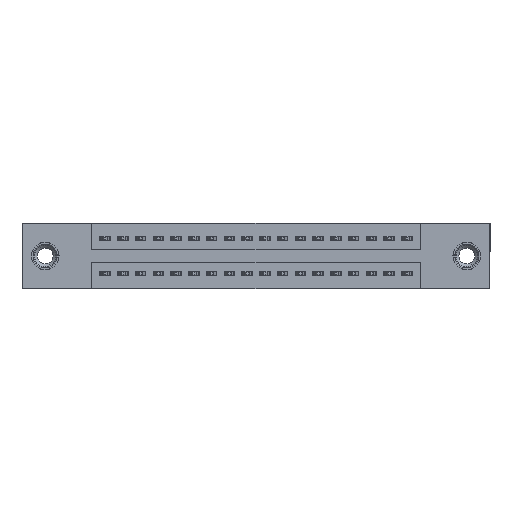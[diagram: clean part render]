
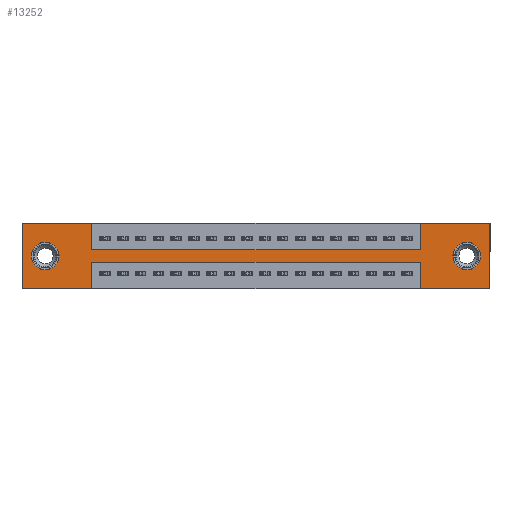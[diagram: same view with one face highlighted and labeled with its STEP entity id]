
A CAD part, front view. The second image highlights one B-rep face of the part: STEP entity #13252.
In plain terms, the highlighted planar face has unit normal (0, -1, 0).
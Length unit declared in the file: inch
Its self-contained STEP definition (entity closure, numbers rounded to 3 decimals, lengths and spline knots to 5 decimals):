
#41 = EDGE_LOOP ( 'NONE', ( #4780, #4870, #1820, #1721, #2063, #2196, #6048, #524, #962, #1680, #601, #4953 ) ) ;
#108 = EDGE_LOOP ( 'NONE', ( #6852, #15139 ) ) ;
#152 = VECTOR ( 'NONE', #4860, 39.37008 ) ;
#318 = CARTESIAN_POINT ( 'NONE',  ( 2.635, 0., -0.37 ) ) ;
#524 = ORIENTED_EDGE ( 'NONE', *, *, #14031, .F. ) ;
#582 = LINE ( 'NONE', #17118, #8273 ) ;
#601 = ORIENTED_EDGE ( 'NONE', *, *, #5658, .F. ) ;
#962 = ORIENTED_EDGE ( 'NONE', *, *, #12562, .F. ) ;
#1312 = CARTESIAN_POINT ( 'NONE',  ( 0.3925, 0., -0.37 ) ) ;
#1385 = DIRECTION ( 'NONE',  ( 0., 0., -1. ) ) ;
#1387 = DIRECTION ( 'NONE',  ( 0., 0., -1. ) ) ;
#1504 = DIRECTION ( 'NONE',  ( 0., 0., -1. ) ) ;
#1521 = DIRECTION ( 'NONE',  ( -1., 0., 0. ) ) ;
#1533 = VECTOR ( 'NONE', #14703, 39.37008 ) ;
#1588 = CIRCLE ( 'NONE', #16197, 0.078 ) ;
#1680 = ORIENTED_EDGE ( 'NONE', *, *, #13107, .F. ) ;
#1721 = ORIENTED_EDGE ( 'NONE', *, *, #17883, .F. ) ;
#1820 = ORIENTED_EDGE ( 'NONE', *, *, #15343, .F. ) ;
#1872 = CARTESIAN_POINT ( 'NONE',  ( 0., 0., 0. ) ) ;
#2063 = ORIENTED_EDGE ( 'NONE', *, *, #8920, .F. ) ;
#2196 = ORIENTED_EDGE ( 'NONE', *, *, #2887, .F. ) ;
#2735 = VERTEX_POINT ( 'NONE', #13719 ) ;
#2766 = DIRECTION ( 'NONE',  ( 1., 0., 0. ) ) ;
#2886 = VECTOR ( 'NONE', #1521, 39.37008 ) ;
#2887 = EDGE_CURVE ( 'NONE', #11552, #13812, #14918, .T. ) ;
#3115 = EDGE_LOOP ( 'NONE', ( #5435, #9566 ) ) ;
#3191 = EDGE_CURVE ( 'NONE', #7550, #15297, #17649, .T. ) ;
#3318 = VECTOR ( 'NONE', #1504, 39.37008 ) ;
#3362 = VERTEX_POINT ( 'NONE', #9424 ) ;
#3651 = CARTESIAN_POINT ( 'NONE',  ( 0.13, 0., -0.185 ) ) ;
#3683 = CARTESIAN_POINT ( 'NONE',  ( 0., 0., -0.37 ) ) ;
#4094 = VERTEX_POINT ( 'NONE', #15464 ) ;
#4113 = CARTESIAN_POINT ( 'NONE',  ( 0., 0., 0. ) ) ;
#4128 = VERTEX_POINT ( 'NONE', #14123 ) ;
#4216 = AXIS2_PLACEMENT_3D ( 'NONE', #10739, #6169, #16668 ) ;
#4217 = CARTESIAN_POINT ( 'NONE',  ( 2.635, 0., 0. ) ) ;
#4353 = CARTESIAN_POINT ( 'NONE',  ( 2.635, 0., 0. ) ) ;
#4401 = CARTESIAN_POINT ( 'NONE',  ( 2.2425, 0., -0.22 ) ) ;
#4633 = PLANE ( 'NONE',  #4216 ) ;
#4780 = ORIENTED_EDGE ( 'NONE', *, *, #16387, .F. ) ;
#4860 = DIRECTION ( 'NONE',  ( 1., 0., 0. ) ) ;
#4870 = ORIENTED_EDGE ( 'NONE', *, *, #10875, .F. ) ;
#4953 = ORIENTED_EDGE ( 'NONE', *, *, #16055, .F. ) ;
#5014 = CARTESIAN_POINT ( 'NONE',  ( 2.505, 0., -0.107 ) ) ;
#5093 = VERTEX_POINT ( 'NONE', #4401 ) ;
#5167 = DIRECTION ( 'NONE',  ( 0., 0., 1. ) ) ;
#5435 = ORIENTED_EDGE ( 'NONE', *, *, #14413, .T. ) ;
#5601 = LINE ( 'NONE', #4113, #1533 ) ;
#5604 = AXIS2_PLACEMENT_3D ( 'NONE', #8463, #18890, #10000 ) ;
#5658 = EDGE_CURVE ( 'NONE', #4128, #2735, #5601, .T. ) ;
#5840 = CARTESIAN_POINT ( 'NONE',  ( 0., 0., 0. ) ) ;
#5999 = CARTESIAN_POINT ( 'NONE',  ( 0.3925, 0., -0.37 ) ) ;
#6048 = ORIENTED_EDGE ( 'NONE', *, *, #18823, .F. ) ;
#6169 = DIRECTION ( 'NONE',  ( 0., -1., 0. ) ) ;
#6553 = VECTOR ( 'NONE', #11298, 39.37008 ) ;
#6793 = DIRECTION ( 'NONE',  ( 0., 0., 1. ) ) ;
#6852 = ORIENTED_EDGE ( 'NONE', *, *, #9925, .T. ) ;
#7401 = LINE ( 'NONE', #13758, #3318 ) ;
#7550 = VERTEX_POINT ( 'NONE', #8670 ) ;
#7720 = CARTESIAN_POINT ( 'NONE',  ( 2.2425, 0., -0.15 ) ) ;
#8029 = AXIS2_PLACEMENT_3D ( 'NONE', #3651, #14250, #5167 ) ;
#8048 = CARTESIAN_POINT ( 'NONE',  ( 0.3925, 0., -0.15 ) ) ;
#8273 = VECTOR ( 'NONE', #18610, 39.37008 ) ;
#8451 = VERTEX_POINT ( 'NONE', #7720 ) ;
#8463 = CARTESIAN_POINT ( 'NONE',  ( 0.13, 0., -0.185 ) ) ;
#8566 = VERTEX_POINT ( 'NONE', #318 ) ;
#8630 = LINE ( 'NONE', #4217, #16094 ) ;
#8670 = CARTESIAN_POINT ( 'NONE',  ( 2.505, 0., -0.263 ) ) ;
#8920 = EDGE_CURVE ( 'NONE', #13812, #8566, #8630, .T. ) ;
#8936 = VECTOR ( 'NONE', #17997, 39.37008 ) ;
#9291 = VERTEX_POINT ( 'NONE', #18512 ) ;
#9424 = CARTESIAN_POINT ( 'NONE',  ( 0.13, 0., -0.263 ) ) ;
#9535 = VERTEX_POINT ( 'NONE', #17654 ) ;
#9566 = ORIENTED_EDGE ( 'NONE', *, *, #3191, .T. ) ;
#9925 = EDGE_CURVE ( 'NONE', #13351, #3362, #17680, .T. ) ;
#10000 = DIRECTION ( 'NONE',  ( 0., 0., 1. ) ) ;
#10570 = DIRECTION ( 'NONE',  ( 0., 1., 0. ) ) ;
#10578 = DIRECTION ( 'NONE',  ( 0., 1., 0. ) ) ;
#10726 = FACE_OUTER_BOUND ( 'NONE', #41, .T. ) ;
#10739 = CARTESIAN_POINT ( 'NONE',  ( 0., 0., -0.37 ) ) ;
#10875 = EDGE_CURVE ( 'NONE', #5093, #9535, #18335, .T. ) ;
#10974 = VECTOR ( 'NONE', #15568, 39.37008 ) ;
#11298 = DIRECTION ( 'NONE',  ( -1., 0., 0. ) ) ;
#11336 = CARTESIAN_POINT ( 'NONE',  ( 2.2425, 0., 0. ) ) ;
#11552 = VERTEX_POINT ( 'NONE', #12689 ) ;
#11661 = FACE_BOUND ( 'NONE', #3115, .T. ) ;
#11693 = AXIS2_PLACEMENT_3D ( 'NONE', #19442, #10578, #1387 ) ;
#12371 = LINE ( 'NONE', #16898, #152 ) ;
#12562 = EDGE_CURVE ( 'NONE', #9291, #19414, #7401, .T. ) ;
#12689 = CARTESIAN_POINT ( 'NONE',  ( 2.2425, 0., 0. ) ) ;
#12871 = EDGE_CURVE ( 'NONE', #3362, #13351, #14227, .T. ) ;
#12968 = LINE ( 'NONE', #5999, #8936 ) ;
#13107 = EDGE_CURVE ( 'NONE', #2735, #9291, #13534, .T. ) ;
#13215 = VECTOR ( 'NONE', #6793, 39.37008 ) ;
#13252 = ADVANCED_FACE ( 'NONE', ( #11661, #14670, #10726 ), #4633, .T. ) ;
#13351 = VERTEX_POINT ( 'NONE', #18345 ) ;
#13534 = LINE ( 'NONE', #5840, #17429 ) ;
#13719 = CARTESIAN_POINT ( 'NONE',  ( 0., 0., 0. ) ) ;
#13758 = CARTESIAN_POINT ( 'NONE',  ( 0.3925, 0., 0. ) ) ;
#13812 = VERTEX_POINT ( 'NONE', #4353 ) ;
#14031 = EDGE_CURVE ( 'NONE', #19414, #8451, #12371, .T. ) ;
#14123 = CARTESIAN_POINT ( 'NONE',  ( 0., 0., -0.37 ) ) ;
#14227 = CIRCLE ( 'NONE', #5604, 0.078 ) ;
#14250 = DIRECTION ( 'NONE',  ( 0., 1., 0. ) ) ;
#14390 = VERTEX_POINT ( 'NONE', #1312 ) ;
#14413 = EDGE_CURVE ( 'NONE', #15297, #7550, #1588, .T. ) ;
#14670 = FACE_BOUND ( 'NONE', #108, .T. ) ;
#14703 = DIRECTION ( 'NONE',  ( 0., 0., 1. ) ) ;
#14807 = DIRECTION ( 'NONE',  ( 0., 0., -1. ) ) ;
#14918 = LINE ( 'NONE', #1872, #10974 ) ;
#15139 = ORIENTED_EDGE ( 'NONE', *, *, #12871, .T. ) ;
#15297 = VERTEX_POINT ( 'NONE', #5014 ) ;
#15343 = EDGE_CURVE ( 'NONE', #4094, #5093, #582, .T. ) ;
#15423 = LINE ( 'NONE', #16643, #2886 ) ;
#15464 = CARTESIAN_POINT ( 'NONE',  ( 2.2425, 0., -0.37 ) ) ;
#15568 = DIRECTION ( 'NONE',  ( 1., 0., 0. ) ) ;
#16055 = EDGE_CURVE ( 'NONE', #14390, #4128, #18487, .T. ) ;
#16094 = VECTOR ( 'NONE', #14807, 39.37008 ) ;
#16197 = AXIS2_PLACEMENT_3D ( 'NONE', #19437, #10570, #1385 ) ;
#16387 = EDGE_CURVE ( 'NONE', #9535, #14390, #12968, .T. ) ;
#16643 = CARTESIAN_POINT ( 'NONE',  ( 0., 0., -0.37 ) ) ;
#16668 = DIRECTION ( 'NONE',  ( 0., 0., -1. ) ) ;
#16898 = CARTESIAN_POINT ( 'NONE',  ( 0.3925, 0., -0.15 ) ) ;
#17102 = LINE ( 'NONE', #11336, #13215 ) ;
#17118 = CARTESIAN_POINT ( 'NONE',  ( 2.2425, 0., -0.37 ) ) ;
#17128 = CARTESIAN_POINT ( 'NONE',  ( 0.3925, 0., -0.22 ) ) ;
#17429 = VECTOR ( 'NONE', #2766, 39.37008 ) ;
#17649 = CIRCLE ( 'NONE', #11693, 0.078 ) ;
#17654 = CARTESIAN_POINT ( 'NONE',  ( 0.3925, 0., -0.22 ) ) ;
#17680 = CIRCLE ( 'NONE', #8029, 0.078 ) ;
#17883 = EDGE_CURVE ( 'NONE', #8566, #4094, #15423, .T. ) ;
#17997 = DIRECTION ( 'NONE',  ( 0., 0., -1. ) ) ;
#18335 = LINE ( 'NONE', #17128, #18806 ) ;
#18345 = CARTESIAN_POINT ( 'NONE',  ( 0.13, 0., -0.107 ) ) ;
#18487 = LINE ( 'NONE', #3683, #6553 ) ;
#18512 = CARTESIAN_POINT ( 'NONE',  ( 0.3925, 0., 0. ) ) ;
#18610 = DIRECTION ( 'NONE',  ( 0., 0., 1. ) ) ;
#18624 = DIRECTION ( 'NONE',  ( -1., 0., 0. ) ) ;
#18806 = VECTOR ( 'NONE', #18624, 39.37008 ) ;
#18823 = EDGE_CURVE ( 'NONE', #8451, #11552, #17102, .T. ) ;
#18890 = DIRECTION ( 'NONE',  ( 0., 1., 0. ) ) ;
#19414 = VERTEX_POINT ( 'NONE', #8048 ) ;
#19437 = CARTESIAN_POINT ( 'NONE',  ( 2.505, 0., -0.185 ) ) ;
#19442 = CARTESIAN_POINT ( 'NONE',  ( 2.505, 0., -0.185 ) ) ;
